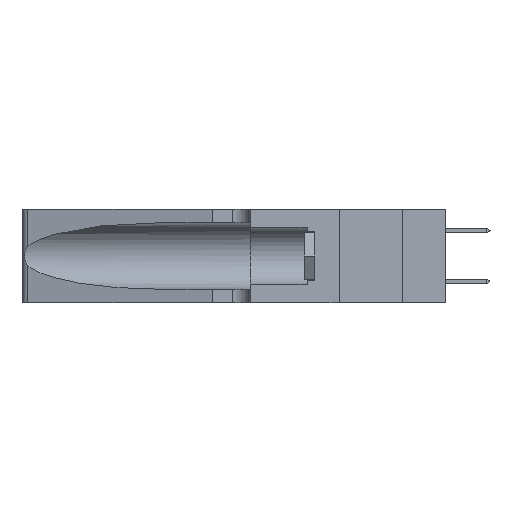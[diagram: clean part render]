
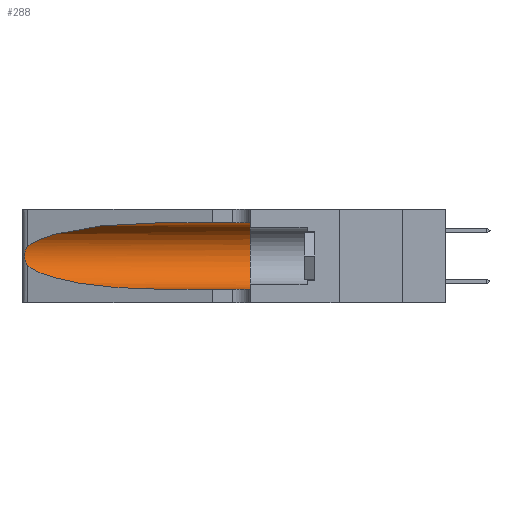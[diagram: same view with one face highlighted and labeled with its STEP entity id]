
A CAD part, left-side view. The second image highlights one B-rep face of the part: STEP entity #288.
In plain terms, the highlighted cylindrical face has radius 3.308 mm (diameter 6.617 mm), a partial arc.
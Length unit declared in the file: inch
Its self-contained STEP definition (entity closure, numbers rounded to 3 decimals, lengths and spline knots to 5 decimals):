
#107 = VECTOR ( 'NONE', #3200, 39.37008 ) ;
#224 = CARTESIAN_POINT ( 'NONE',  ( 0.1305, 0.35, 0.31525 ) ) ;
#288 = ADVANCED_FACE ( 'NONE', ( #4683 ), #27536, .F. ) ;
#489 = ORIENTED_EDGE ( 'NONE', *, *, #3583, .T. ) ;
#512 = VERTEX_POINT ( 'NONE', #224 ) ;
#682 = VERTEX_POINT ( 'NONE', #12035 ) ;
#1417 = DIRECTION ( 'NONE',  ( 0., -1., 0. ) ) ;
#1467 = EDGE_CURVE ( 'NONE', #18796, #512, #19448, .T. ) ;
#1512 = CARTESIAN_POINT ( 'NONE',  ( 0.2373, 1.15595, 0.08982 ) ) ;
#2596 = AXIS2_PLACEMENT_3D ( 'NONE', #12500, #28424, #25942 ) ;
#2607 = VERTEX_POINT ( 'NONE', #8790 ) ;
#2643 = EDGE_LOOP ( 'NONE', ( #11393, #489, #3451, #24295, #11241, #23711 ) ) ;
#2748 = CARTESIAN_POINT ( 'NONE',  ( 0.18966, 0.96281, 0.31525 ) ) ;
#3200 = DIRECTION ( 'NONE',  ( 0., -1., 0. ) ) ;
#3260 = AXIS2_PLACEMENT_3D ( 'NONE', #25724, #21420, #12173 ) ;
#3451 = ORIENTED_EDGE ( 'NONE', *, *, #6537, .T. ) ;
#3525 = CARTESIAN_POINT ( 'NONE',  ( 0.25856, 1.23593, 0.16098 ) ) ;
#3583 = EDGE_CURVE ( 'NONE', #27267, #682, #22498, .T. ) ;
#3634 = CARTESIAN_POINT ( 'NONE',  ( 0.25639, 1.23186, 0.15144 ) ) ;
#4683 = FACE_OUTER_BOUND ( 'NONE', #2643, .T. ) ;
#4958 = CARTESIAN_POINT ( 'NONE',  ( 0.1305, 0.72297, 0.31525 ) ) ;
#5725 = CARTESIAN_POINT ( 'NONE',  ( 0.25487, 1.22718, 0.14631 ) ) ;
#6107 = CIRCLE ( 'NONE', #3260, 0.13025 ) ;
#6537 = EDGE_CURVE ( 'NONE', #682, #2607, #8801, .T. ) ;
#7270 = CARTESIAN_POINT ( 'NONE',  ( 0.2373, 1.15595, 0.28018 ) ) ;
#7706 = CARTESIAN_POINT ( 'NONE',  ( 0.26075, 1.23896, 0.178 ) ) ;
#8316 = CARTESIAN_POINT ( 'NONE',  ( 0.25789, 1.23486, 0.15765 ) ) ;
#8790 = CARTESIAN_POINT ( 'NONE',  ( 0.1305, 0.72297, 0.05475 ) ) ;
#8801 =( BOUNDED_CURVE ( )  B_SPLINE_CURVE ( 3, ( #17836, #1512, #26888, #18031 ),
 .UNSPECIFIED., .F., .T. ) 
 B_SPLINE_CURVE_WITH_KNOTS ( ( 4, 4 ),
 ( 3.44316, 4.71239 ),
 .UNSPECIFIED. ) 
 CURVE ( )  GEOMETRIC_REPRESENTATION_ITEM ( )  RATIONAL_B_SPLINE_CURVE ( ( 1., 0.87, 0.87, 1. ) ) 
 REPRESENTATION_ITEM ( '' )  );
#9801 = CARTESIAN_POINT ( 'NONE',  ( 0.1305, 0.72297, 0.31525 ) ) ;
#10775 = CARTESIAN_POINT ( 'NONE',  ( 0.25555, 1.22994, 0.2215 ) ) ;
#11241 = ORIENTED_EDGE ( 'NONE', *, *, #23844, .F. ) ;
#11393 = ORIENTED_EDGE ( 'NONE', *, *, #23377, .T. ) ;
#12035 = CARTESIAN_POINT ( 'NONE',  ( 0.25487, 1.22718, 0.14631 ) ) ;
#12173 = DIRECTION ( 'NONE',  ( 0., 0., 1. ) ) ;
#12500 = CARTESIAN_POINT ( 'NONE',  ( 0.1305, 1.61858, 0.185 ) ) ;
#13849 = CARTESIAN_POINT ( 'NONE',  ( 0.26075, 1.23896, 0.19203 ) ) ;
#14872 = VECTOR ( 'NONE', #1417, 39.37008 ) ;
#15003 = VERTEX_POINT ( 'NONE', #23130 ) ;
#15102 =( BOUNDED_CURVE ( )  B_SPLINE_CURVE ( 3, ( #4958, #2748, #7270, #23113 ),
 .UNSPECIFIED., .F., .F. ) 
 B_SPLINE_CURVE_WITH_KNOTS ( ( 4, 4 ),
 ( 1.5708, 2.84003 ),
 .UNSPECIFIED. ) 
 CURVE ( )  GEOMETRIC_REPRESENTATION_ITEM ( )  RATIONAL_B_SPLINE_CURVE ( ( 1., 0.87, 0.87, 1. ) ) 
 REPRESENTATION_ITEM ( '' )  );
#15164 = CARTESIAN_POINT ( 'NONE',  ( 0.26017, 1.23833, 0.17102 ) ) ;
#15490 = CARTESIAN_POINT ( 'NONE',  ( 0.25639, 1.23184, 0.21858 ) ) ;
#17836 = CARTESIAN_POINT ( 'NONE',  ( 0.25487, 1.22718, 0.14631 ) ) ;
#18031 = CARTESIAN_POINT ( 'NONE',  ( 0.1305, 0.72297, 0.05475 ) ) ;
#18796 = VERTEX_POINT ( 'NONE', #9801 ) ;
#19448 = LINE ( 'NONE', #26492, #14872 ) ;
#19811 = CARTESIAN_POINT ( 'NONE',  ( 0.25487, 1.22718, 0.22369 ) ) ;
#20841 = EDGE_CURVE ( 'NONE', #2607, #15003, #26207, .T. ) ;
#21420 = DIRECTION ( 'NONE',  ( 0., 1., 0. ) ) ;
#21564 = CARTESIAN_POINT ( 'NONE',  ( 0.25555, 1.22993, 0.14849 ) ) ;
#22498 = B_SPLINE_CURVE_WITH_KNOTS ( 'NONE', 3,
 ( #19811, #10775, #15490, #24613, #25085, #23172, #13849, #7706, #15164, #3525, #8316, #3634, #21564, #5725 ),
 .UNSPECIFIED., .F., .F.,
 ( 4, 2, 2, 2, 2, 2, 4 ),
 ( 0., 0.00027, 0.00053, 0.00107, 0.0016, 0.00187, 0.00214 ),
 .UNSPECIFIED. ) ;
#22837 = CARTESIAN_POINT ( 'NONE',  ( 0.25487, 1.22718, 0.22369 ) ) ;
#23113 = CARTESIAN_POINT ( 'NONE',  ( 0.25487, 1.22718, 0.22369 ) ) ;
#23130 = CARTESIAN_POINT ( 'NONE',  ( 0.1305, 0.35, 0.05475 ) ) ;
#23172 = CARTESIAN_POINT ( 'NONE',  ( 0.26018, 1.23835, 0.19895 ) ) ;
#23377 = EDGE_CURVE ( 'NONE', #18796, #27267, #15102, .T. ) ;
#23711 = ORIENTED_EDGE ( 'NONE', *, *, #1467, .F. ) ;
#23766 = CARTESIAN_POINT ( 'NONE',  ( 0.1305, 1.61858, 0.05475 ) ) ;
#23844 = EDGE_CURVE ( 'NONE', #512, #15003, #6107, .T. ) ;
#24295 = ORIENTED_EDGE ( 'NONE', *, *, #20841, .T. ) ;
#24613 = CARTESIAN_POINT ( 'NONE',  ( 0.25787, 1.23484, 0.2124 ) ) ;
#25085 = CARTESIAN_POINT ( 'NONE',  ( 0.25854, 1.2359, 0.20912 ) ) ;
#25724 = CARTESIAN_POINT ( 'NONE',  ( 0.1305, 0.35, 0.185 ) ) ;
#25942 = DIRECTION ( 'NONE',  ( 0., 0., -1. ) ) ;
#26207 = LINE ( 'NONE', #23766, #107 ) ;
#26492 = CARTESIAN_POINT ( 'NONE',  ( 0.1305, 1.61858, 0.31525 ) ) ;
#26888 = CARTESIAN_POINT ( 'NONE',  ( 0.18966, 0.96281, 0.05475 ) ) ;
#27267 = VERTEX_POINT ( 'NONE', #22837 ) ;
#27536 = CYLINDRICAL_SURFACE ( 'NONE', #2596, 0.13025 ) ;
#28424 = DIRECTION ( 'NONE',  ( 0., -1., 0. ) ) ;
